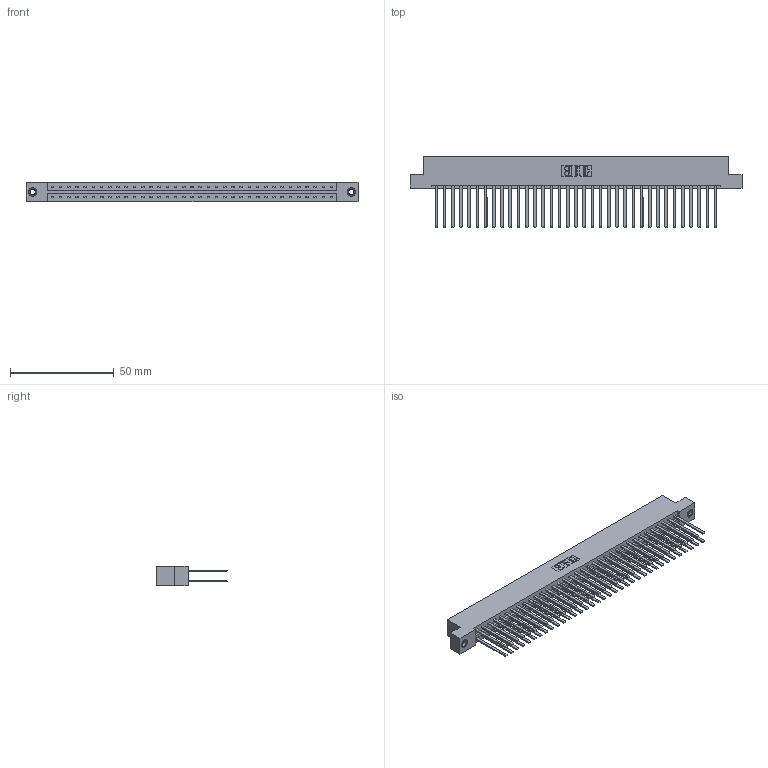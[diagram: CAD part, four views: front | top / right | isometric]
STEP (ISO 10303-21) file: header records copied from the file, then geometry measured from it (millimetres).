
FILE_DESCRIPTION (( 'STEP AP203' ), '1' );
FILE_NAME ('833-070-544-207.STEP', '2020-06-05T12:44:53', ( '' ), ( '' ), 'SwSTEP 2.0', 'SolidWorks 2020', '' );
FILE_SCHEMA (( 'CONFIG_CONTROL_DESIGN' ));
Length unit declared in the file: inch
Products named in the file (4): 833 Part_Flush - .156 Dia - TI; 345-250-001_345-250-005-103; 833-070-544-207; 345-292-001_345-293-144
Assembly tree (73 placements, depth 2):
  833-070-544-207
    833 Part_Flush - .156 Dia - TI
    345-292-001_345-293-144  x70
    345-250-001_345-250-005-103  x2
Bounding box: 160.22 x 34.3 x 9.4 mm (x, y, z)
Volume: 17260.2 mm3; surface area: 23524.2 mm2
Topology: 73 solids, 73 shells, 3394 faces, 10037 edges, 6590 vertices
Faces by surface type: plane 2342, cylinder 1036, cone 12, torus 4
Entity records: 24424 total; most frequent: CARTESIAN_POINT 4037, ORIENTED_EDGE 3966, DIRECTION 3489, EDGE_CURVE 1983, LINE 1839, VECTOR 1839, VERTEX_POINT 1316, AXIS2_PLACEMENT_3D 825
